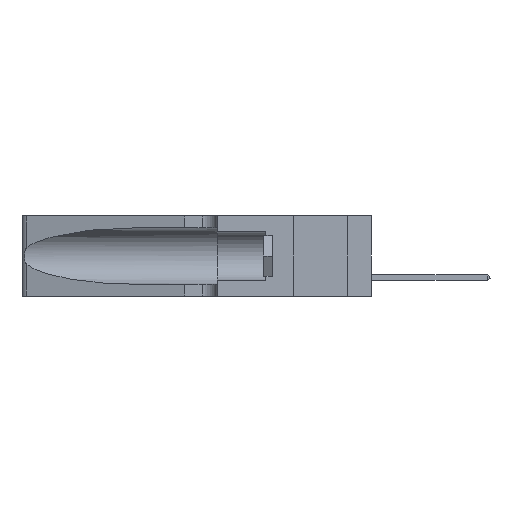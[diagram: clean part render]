
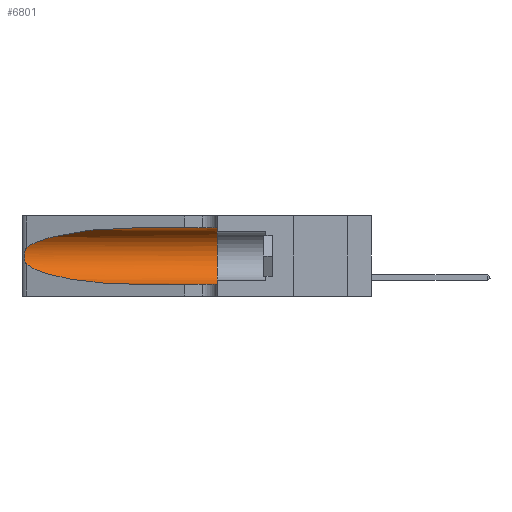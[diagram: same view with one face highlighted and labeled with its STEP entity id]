
A CAD part, left-side view. The second image highlights one B-rep face of the part: STEP entity #6801.
In plain terms, the highlighted cylindrical face has radius 3.308 mm (diameter 6.617 mm), a partial arc.
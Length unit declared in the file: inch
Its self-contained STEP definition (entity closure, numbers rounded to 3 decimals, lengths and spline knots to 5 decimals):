
#401 = DIRECTION ( 'NONE',  ( 0., -1., 0. ) ) ;
#646 = VERTEX_POINT ( 'NONE', #1048 ) ;
#1002 = ORIENTED_EDGE ( 'NONE', *, *, #7424, .F. ) ;
#1048 = CARTESIAN_POINT ( 'NONE',  ( 0.1305, 0.35, 0.31525 ) ) ;
#1056 = EDGE_LOOP ( 'NONE', ( #21603, #6790, #20829, #15243, #1002, #11056 ) ) ;
#1060 = CARTESIAN_POINT ( 'NONE',  ( 0.1305, 0.72297, 0.05475 ) ) ;
#1782 = CARTESIAN_POINT ( 'NONE',  ( 0.1305, 0.35, 0.185 ) ) ;
#3209 = CARTESIAN_POINT ( 'NONE',  ( 0.18966, 0.96281, 0.31525 ) ) ;
#3642 = CARTESIAN_POINT ( 'NONE',  ( 0.26017, 1.23833, 0.17102 ) ) ;
#3714 = VECTOR ( 'NONE', #8600, 39.37008 ) ;
#3883 = CARTESIAN_POINT ( 'NONE',  ( 0.26018, 1.23835, 0.19895 ) ) ;
#4027 = CARTESIAN_POINT ( 'NONE',  ( 0.25487, 1.22718, 0.14631 ) ) ;
#4272 = EDGE_CURVE ( 'NONE', #16016, #20876, #18444, .T. ) ;
#4535 = CARTESIAN_POINT ( 'NONE',  ( 0.1305, 1.61858, 0.185 ) ) ;
#5504 = CARTESIAN_POINT ( 'NONE',  ( 0.25639, 1.23186, 0.15144 ) ) ;
#5984 = CARTESIAN_POINT ( 'NONE',  ( 0.2373, 1.15595, 0.08982 ) ) ;
#6596 = DIRECTION ( 'NONE',  ( 0., -1., 0. ) ) ;
#6640 = CIRCLE ( 'NONE', #6985, 0.13025 ) ;
#6790 = ORIENTED_EDGE ( 'NONE', *, *, #10258, .T. ) ;
#6801 = ADVANCED_FACE ( 'NONE', ( #11288 ), #21673, .F. ) ;
#6985 = AXIS2_PLACEMENT_3D ( 'NONE', #1782, #22194, #14795 ) ;
#7256 = CARTESIAN_POINT ( 'NONE',  ( 0.26075, 1.23896, 0.178 ) ) ;
#7403 = CARTESIAN_POINT ( 'NONE',  ( 0.25487, 1.22718, 0.14631 ) ) ;
#7424 = EDGE_CURVE ( 'NONE', #646, #10352, #6640, .T. ) ;
#7819 = EDGE_CURVE ( 'NONE', #20260, #646, #23744, .T. ) ;
#8600 = DIRECTION ( 'NONE',  ( 0., -1., 0. ) ) ;
#9435 = CARTESIAN_POINT ( 'NONE',  ( 0.25639, 1.23184, 0.21858 ) ) ;
#10258 = EDGE_CURVE ( 'NONE', #14917, #16016, #14196, .T. ) ;
#10352 = VERTEX_POINT ( 'NONE', #22101 ) ;
#10509 = CARTESIAN_POINT ( 'NONE',  ( 0.1305, 0.72297, 0.31525 ) ) ;
#10985 = CARTESIAN_POINT ( 'NONE',  ( 0.25789, 1.23486, 0.15765 ) ) ;
#11056 = ORIENTED_EDGE ( 'NONE', *, *, #7819, .F. ) ;
#11065 = CARTESIAN_POINT ( 'NONE',  ( 0.26075, 1.23896, 0.19203 ) ) ;
#11215 = CARTESIAN_POINT ( 'NONE',  ( 0.25787, 1.23484, 0.2124 ) ) ;
#11288 = FACE_OUTER_BOUND ( 'NONE', #1056, .T. ) ;
#11743 = EDGE_CURVE ( 'NONE', #20876, #10352, #22642, .T. ) ;
#13539 = CARTESIAN_POINT ( 'NONE',  ( 0.18966, 0.96281, 0.05475 ) ) ;
#14196 = B_SPLINE_CURVE_WITH_KNOTS ( 'NONE', 3,
 ( #20446, #23983, #9435, #11215, #22074, #3883, #11065, #7256, #3642, #16613, #10985, #5504, #18460, #7403 ),
 .UNSPECIFIED., .F., .F.,
 ( 4, 2, 2, 2, 2, 2, 4 ),
 ( 0., 0.00027, 0.00053, 0.00107, 0.0016, 0.00187, 0.00214 ),
 .UNSPECIFIED. ) ;
#14795 = DIRECTION ( 'NONE',  ( 0., 0., 1. ) ) ;
#14917 = VERTEX_POINT ( 'NONE', #21306 ) ;
#15150 = CARTESIAN_POINT ( 'NONE',  ( 0.25487, 1.22718, 0.14631 ) ) ;
#15243 = ORIENTED_EDGE ( 'NONE', *, *, #11743, .T. ) ;
#16016 = VERTEX_POINT ( 'NONE', #4027 ) ;
#16040 = CARTESIAN_POINT ( 'NONE',  ( 0.1305, 1.61858, 0.31525 ) ) ;
#16613 = CARTESIAN_POINT ( 'NONE',  ( 0.25856, 1.23593, 0.16098 ) ) ;
#16861 = VECTOR ( 'NONE', #401, 39.37008 ) ;
#16920 = CARTESIAN_POINT ( 'NONE',  ( 0.1305, 0.72297, 0.05475 ) ) ;
#17589 = DIRECTION ( 'NONE',  ( 0., 0., -1. ) ) ;
#18444 =( BOUNDED_CURVE ( )  B_SPLINE_CURVE ( 3, ( #15150, #5984, #13539, #16920 ),
 .UNSPECIFIED., .F., .T. ) 
 B_SPLINE_CURVE_WITH_KNOTS ( ( 4, 4 ),
 ( 3.44316, 4.71239 ),
 .UNSPECIFIED. ) 
 CURVE ( )  GEOMETRIC_REPRESENTATION_ITEM ( )  RATIONAL_B_SPLINE_CURVE ( ( 1., 0.87, 0.87, 1. ) ) 
 REPRESENTATION_ITEM ( '' )  );
#18460 = CARTESIAN_POINT ( 'NONE',  ( 0.25555, 1.22993, 0.14849 ) ) ;
#18801 = EDGE_CURVE ( 'NONE', #20260, #14917, #23946, .T. ) ;
#20091 = CARTESIAN_POINT ( 'NONE',  ( 0.2373, 1.15595, 0.28018 ) ) ;
#20164 = CARTESIAN_POINT ( 'NONE',  ( 0.25487, 1.22718, 0.22369 ) ) ;
#20260 = VERTEX_POINT ( 'NONE', #22216 ) ;
#20446 = CARTESIAN_POINT ( 'NONE',  ( 0.25487, 1.22718, 0.22369 ) ) ;
#20829 = ORIENTED_EDGE ( 'NONE', *, *, #4272, .T. ) ;
#20876 = VERTEX_POINT ( 'NONE', #1060 ) ;
#21306 = CARTESIAN_POINT ( 'NONE',  ( 0.25487, 1.22718, 0.22369 ) ) ;
#21603 = ORIENTED_EDGE ( 'NONE', *, *, #18801, .T. ) ;
#21673 = CYLINDRICAL_SURFACE ( 'NONE', #24012, 0.13025 ) ;
#22074 = CARTESIAN_POINT ( 'NONE',  ( 0.25854, 1.2359, 0.20912 ) ) ;
#22101 = CARTESIAN_POINT ( 'NONE',  ( 0.1305, 0.35, 0.05475 ) ) ;
#22194 = DIRECTION ( 'NONE',  ( 0., 1., 0. ) ) ;
#22216 = CARTESIAN_POINT ( 'NONE',  ( 0.1305, 0.72297, 0.31525 ) ) ;
#22608 = CARTESIAN_POINT ( 'NONE',  ( 0.1305, 1.61858, 0.05475 ) ) ;
#22642 = LINE ( 'NONE', #22608, #16861 ) ;
#23744 = LINE ( 'NONE', #16040, #3714 ) ;
#23946 =( BOUNDED_CURVE ( )  B_SPLINE_CURVE ( 3, ( #10509, #3209, #20091, #20164 ),
 .UNSPECIFIED., .F., .F. ) 
 B_SPLINE_CURVE_WITH_KNOTS ( ( 4, 4 ),
 ( 1.5708, 2.84003 ),
 .UNSPECIFIED. ) 
 CURVE ( )  GEOMETRIC_REPRESENTATION_ITEM ( )  RATIONAL_B_SPLINE_CURVE ( ( 1., 0.87, 0.87, 1. ) ) 
 REPRESENTATION_ITEM ( '' )  );
#23983 = CARTESIAN_POINT ( 'NONE',  ( 0.25555, 1.22994, 0.2215 ) ) ;
#24012 = AXIS2_PLACEMENT_3D ( 'NONE', #4535, #6596, #17589 ) ;
